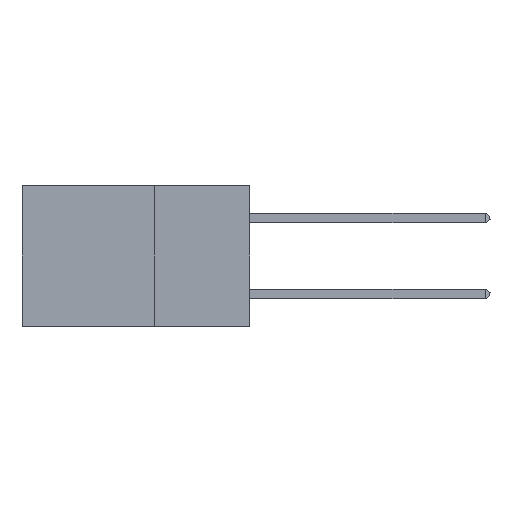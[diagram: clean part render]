
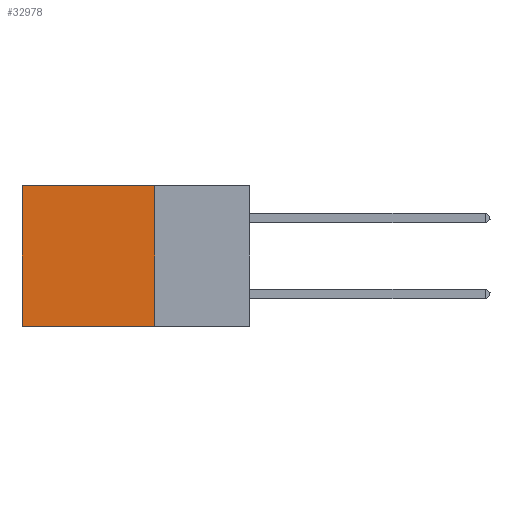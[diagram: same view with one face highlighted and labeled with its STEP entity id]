
A CAD part, left-side view. The second image highlights one B-rep face of the part: STEP entity #32978.
In plain terms, the highlighted planar face has unit normal (-1, 0, 0).
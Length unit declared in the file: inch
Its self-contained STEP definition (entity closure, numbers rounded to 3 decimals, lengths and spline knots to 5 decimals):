
#1262 = AXIS2_PLACEMENT_3D ( 'NONE', #25443, #7751, #28348 ) ;
#1702 = VECTOR ( 'NONE', #10547, 39.37008 ) ;
#2915 = VERTEX_POINT ( 'NONE', #18160 ) ;
#3198 = VERTEX_POINT ( 'NONE', #28140 ) ;
#3504 = EDGE_CURVE ( 'NONE', #2915, #34331, #24816, .T. ) ;
#4835 = LINE ( 'NONE', #14328, #27487 ) ;
#7712 = EDGE_LOOP ( 'NONE', ( #9560, #33900, #23296, #30451 ) ) ;
#7751 = DIRECTION ( 'NONE',  ( 1., 0., 0. ) ) ;
#7787 = CARTESIAN_POINT ( 'NONE',  ( 0.2875, 0.6, -0.37 ) ) ;
#8457 = DIRECTION ( 'NONE',  ( 0., 0., -1. ) ) ;
#8459 = CARTESIAN_POINT ( 'NONE',  ( 0.2875, 0.25, 0. ) ) ;
#9096 = VECTOR ( 'NONE', #17749, 39.37008 ) ;
#9560 = ORIENTED_EDGE ( 'NONE', *, *, #12924, .T. ) ;
#10547 = DIRECTION ( 'NONE',  ( 0., 1., 0. ) ) ;
#12924 = EDGE_CURVE ( 'NONE', #15790, #34331, #4835, .T. ) ;
#13539 = CARTESIAN_POINT ( 'NONE',  ( 0.2875, 0.25, 0. ) ) ;
#14328 = CARTESIAN_POINT ( 'NONE',  ( 0.2875, 0.6, 0. ) ) ;
#14335 = DIRECTION ( 'NONE',  ( 0., 0., -1. ) ) ;
#14786 = CARTESIAN_POINT ( 'NONE',  ( 0.2875, 0.25, -0.37 ) ) ;
#15790 = VERTEX_POINT ( 'NONE', #18671 ) ;
#17569 = LINE ( 'NONE', #13539, #1702 ) ;
#17749 = DIRECTION ( 'NONE',  ( 0., 1., 0. ) ) ;
#18160 = CARTESIAN_POINT ( 'NONE',  ( 0.2875, 0.25, -0.37 ) ) ;
#18671 = CARTESIAN_POINT ( 'NONE',  ( 0.2875, 0.6, 0. ) ) ;
#19539 = PLANE ( 'NONE',  #1262 ) ;
#19739 = FACE_OUTER_BOUND ( 'NONE', #7712, .T. ) ;
#20734 = VECTOR ( 'NONE', #14335, 39.37008 ) ;
#23296 = ORIENTED_EDGE ( 'NONE', *, *, #31855, .F. ) ;
#24816 = LINE ( 'NONE', #14786, #9096 ) ;
#25443 = CARTESIAN_POINT ( 'NONE',  ( 0.2875, 0.25, 0. ) ) ;
#27355 = EDGE_CURVE ( 'NONE', #3198, #15790, #17569, .T. ) ;
#27487 = VECTOR ( 'NONE', #8457, 39.37008 ) ;
#28140 = CARTESIAN_POINT ( 'NONE',  ( 0.2875, 0.25, 0. ) ) ;
#28348 = DIRECTION ( 'NONE',  ( 0., 0., -1. ) ) ;
#29368 = LINE ( 'NONE', #8459, #20734 ) ;
#30451 = ORIENTED_EDGE ( 'NONE', *, *, #27355, .T. ) ;
#31855 = EDGE_CURVE ( 'NONE', #3198, #2915, #29368, .T. ) ;
#32978 = ADVANCED_FACE ( 'NONE', ( #19739 ), #19539, .F. ) ;
#33900 = ORIENTED_EDGE ( 'NONE', *, *, #3504, .F. ) ;
#34331 = VERTEX_POINT ( 'NONE', #7787 ) ;
